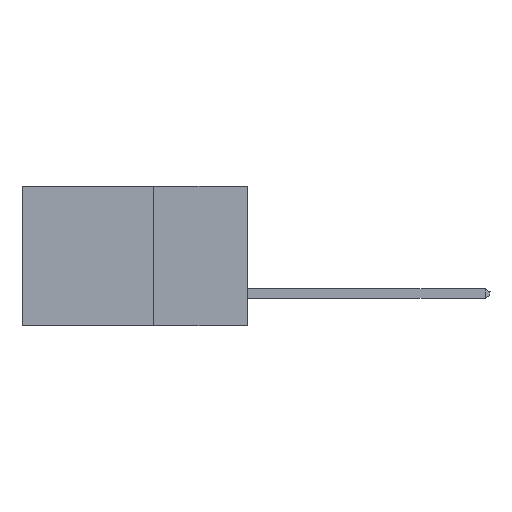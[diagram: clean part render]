
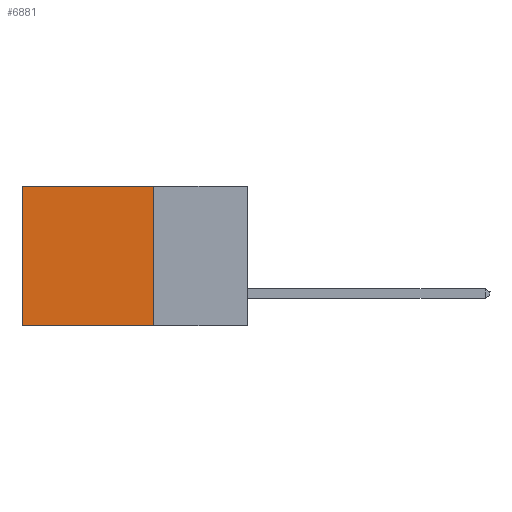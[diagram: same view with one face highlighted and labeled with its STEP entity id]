
A CAD part, left-side view. The second image highlights one B-rep face of the part: STEP entity #6881.
In plain terms, the highlighted planar face has unit normal (-1, 0, 0).
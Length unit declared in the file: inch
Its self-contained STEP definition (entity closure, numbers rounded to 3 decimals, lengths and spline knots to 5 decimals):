
#646 = CARTESIAN_POINT ( 'NONE',  ( 0.2615, 0.25, 0. ) ) ;
#749 = CARTESIAN_POINT ( 'NONE',  ( 0.2615, 0.25, -0.37 ) ) ;
#971 = DIRECTION ( 'NONE',  ( 0., 0., -1. ) ) ;
#1143 = DIRECTION ( 'NONE',  ( 0., 0., -1. ) ) ;
#1755 = EDGE_CURVE ( 'NONE', #2037, #2888, #11204, .T. ) ;
#2037 = VERTEX_POINT ( 'NONE', #3792 ) ;
#2106 = ORIENTED_EDGE ( 'NONE', *, *, #6341, .F. ) ;
#2129 = VERTEX_POINT ( 'NONE', #10250 ) ;
#2349 = EDGE_CURVE ( 'NONE', #2037, #2129, #3522, .T. ) ;
#2888 = VERTEX_POINT ( 'NONE', #749 ) ;
#3025 = DIRECTION ( 'NONE',  ( 0., 0., -1. ) ) ;
#3288 = VECTOR ( 'NONE', #3025, 39.37008 ) ;
#3522 = LINE ( 'NONE', #646, #9357 ) ;
#3760 = VERTEX_POINT ( 'NONE', #9903 ) ;
#3792 = CARTESIAN_POINT ( 'NONE',  ( 0.2615, 0.25, 0. ) ) ;
#3900 = CARTESIAN_POINT ( 'NONE',  ( 0.2615, 0.6, -0.37 ) ) ;
#3925 = VECTOR ( 'NONE', #9704, 39.37008 ) ;
#4022 = EDGE_LOOP ( 'NONE', ( #6265, #2106, #12915, #6806 ) ) ;
#4452 = AXIS2_PLACEMENT_3D ( 'NONE', #11029, #4823, #971 ) ;
#4457 = VECTOR ( 'NONE', #1143, 39.37008 ) ;
#4823 = DIRECTION ( 'NONE',  ( 1., 0., 0. ) ) ;
#5157 = LINE ( 'NONE', #3900, #3288 ) ;
#5646 = CARTESIAN_POINT ( 'NONE',  ( 0.2615, 0.25, -0.37 ) ) ;
#6265 = ORIENTED_EDGE ( 'NONE', *, *, #13141, .T. ) ;
#6341 = EDGE_CURVE ( 'NONE', #2888, #3760, #6763, .T. ) ;
#6763 = LINE ( 'NONE', #5646, #3925 ) ;
#6806 = ORIENTED_EDGE ( 'NONE', *, *, #2349, .T. ) ;
#6881 = ADVANCED_FACE ( 'NONE', ( #9889 ), #11907, .F. ) ;
#7898 = DIRECTION ( 'NONE',  ( 0., 1., 0. ) ) ;
#8254 = CARTESIAN_POINT ( 'NONE',  ( 0.2615, 0.25, -0.37 ) ) ;
#9357 = VECTOR ( 'NONE', #7898, 39.37008 ) ;
#9704 = DIRECTION ( 'NONE',  ( 0., 1., 0. ) ) ;
#9889 = FACE_OUTER_BOUND ( 'NONE', #4022, .T. ) ;
#9903 = CARTESIAN_POINT ( 'NONE',  ( 0.2615, 0.6, -0.37 ) ) ;
#10250 = CARTESIAN_POINT ( 'NONE',  ( 0.2615, 0.6, 0. ) ) ;
#11029 = CARTESIAN_POINT ( 'NONE',  ( 0.2615, 0.25, -0.37 ) ) ;
#11204 = LINE ( 'NONE', #8254, #4457 ) ;
#11907 = PLANE ( 'NONE',  #4452 ) ;
#12915 = ORIENTED_EDGE ( 'NONE', *, *, #1755, .F. ) ;
#13141 = EDGE_CURVE ( 'NONE', #2129, #3760, #5157, .T. ) ;
